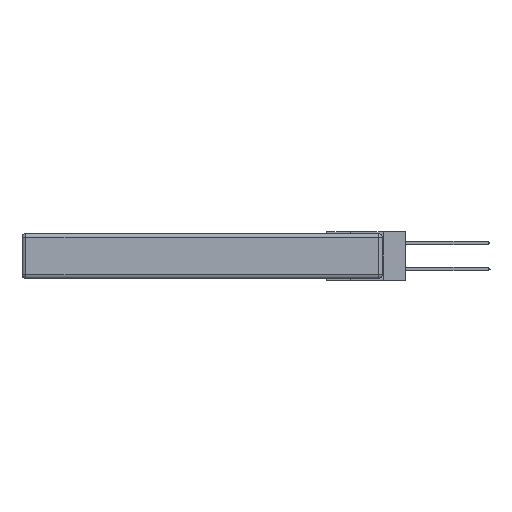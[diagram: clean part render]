
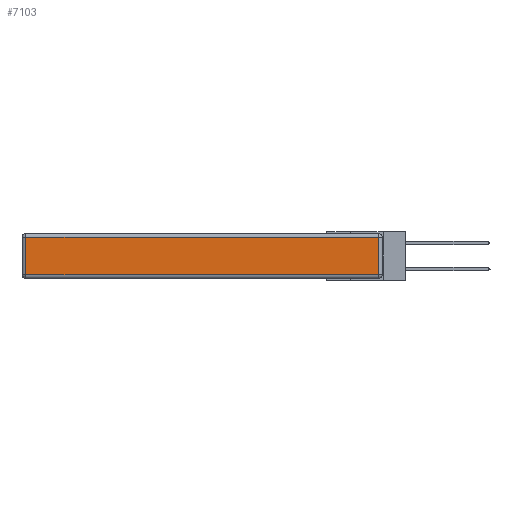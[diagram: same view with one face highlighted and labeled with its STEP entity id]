
A CAD part, left-side view. The second image highlights one B-rep face of the part: STEP entity #7103.
In plain terms, the highlighted planar face has unit normal (-1, 0, 0).
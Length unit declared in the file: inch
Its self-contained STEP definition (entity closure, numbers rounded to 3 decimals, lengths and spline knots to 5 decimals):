
#529 = VECTOR ( 'NONE', #11677, 39.37008 ) ;
#710 = DIRECTION ( 'NONE',  ( -1., 0., 0. ) ) ;
#2430 = CARTESIAN_POINT ( 'NONE',  ( 0., 0., -0.313 ) ) ;
#4632 = FACE_OUTER_BOUND ( 'NONE', #18172, .T. ) ;
#5526 = PLANE ( 'NONE',  #18518 ) ;
#6055 = LINE ( 'NONE', #12053, #23976 ) ;
#6697 = LINE ( 'NONE', #2430, #529 ) ;
#7103 = ADVANCED_FACE ( 'NONE', ( #4632 ), #5526, .T. ) ;
#7314 = EDGE_CURVE ( 'NONE', #27206, #12543, #22209, .T. ) ;
#8073 = ORIENTED_EDGE ( 'NONE', *, *, #9519, .T. ) ;
#9519 = EDGE_CURVE ( 'NONE', #12543, #11149, #16358, .T. ) ;
#10468 = CARTESIAN_POINT ( 'NONE',  ( 0., 2.72, -0.03 ) ) ;
#10956 = CARTESIAN_POINT ( 'NONE',  ( 0., 0.03, -0.343 ) ) ;
#11149 = VERTEX_POINT ( 'NONE', #10468 ) ;
#11677 = DIRECTION ( 'NONE',  ( 0., -1., 0. ) ) ;
#12053 = CARTESIAN_POINT ( 'NONE',  ( 0., 2.72, -0.343 ) ) ;
#12543 = VERTEX_POINT ( 'NONE', #14546 ) ;
#13667 = EDGE_CURVE ( 'NONE', #11149, #14980, #6055, .T. ) ;
#14546 = CARTESIAN_POINT ( 'NONE',  ( 0., 0.03, -0.03 ) ) ;
#14980 = VERTEX_POINT ( 'NONE', #22368 ) ;
#16097 = VECTOR ( 'NONE', #26998, 39.37008 ) ;
#16358 = LINE ( 'NONE', #18600, #27804 ) ;
#16368 = DIRECTION ( 'NONE',  ( 0., 1., 0. ) ) ;
#16875 = DIRECTION ( 'NONE',  ( 0., 0., 1. ) ) ;
#16984 = CARTESIAN_POINT ( 'NONE',  ( 0., 0., -0.343 ) ) ;
#18172 = EDGE_LOOP ( 'NONE', ( #20239, #23080, #8073, #18371 ) ) ;
#18371 = ORIENTED_EDGE ( 'NONE', *, *, #13667, .T. ) ;
#18518 = AXIS2_PLACEMENT_3D ( 'NONE', #16984, #710, #16875 ) ;
#18600 = CARTESIAN_POINT ( 'NONE',  ( 0., 2.75, -0.03 ) ) ;
#20239 = ORIENTED_EDGE ( 'NONE', *, *, #28556, .T. ) ;
#22209 = LINE ( 'NONE', #10956, #16097 ) ;
#22322 = CARTESIAN_POINT ( 'NONE',  ( 0., 0.03, -0.313 ) ) ;
#22368 = CARTESIAN_POINT ( 'NONE',  ( 0., 2.72, -0.313 ) ) ;
#23080 = ORIENTED_EDGE ( 'NONE', *, *, #7314, .T. ) ;
#23976 = VECTOR ( 'NONE', #25993, 39.37008 ) ;
#25993 = DIRECTION ( 'NONE',  ( 0., 0., -1. ) ) ;
#26998 = DIRECTION ( 'NONE',  ( 0., 0., 1. ) ) ;
#27206 = VERTEX_POINT ( 'NONE', #22322 ) ;
#27804 = VECTOR ( 'NONE', #16368, 39.37008 ) ;
#28556 = EDGE_CURVE ( 'NONE', #14980, #27206, #6697, .T. ) ;
